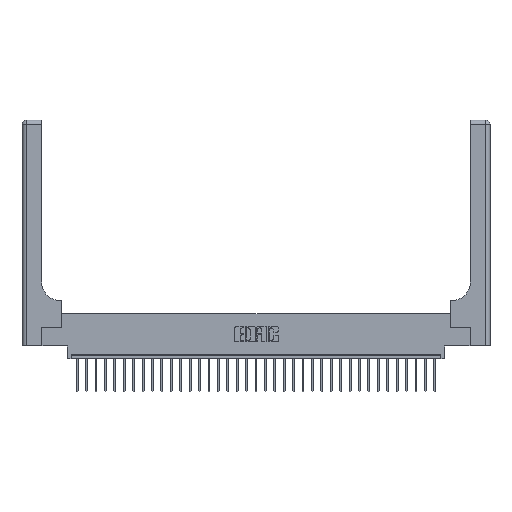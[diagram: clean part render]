
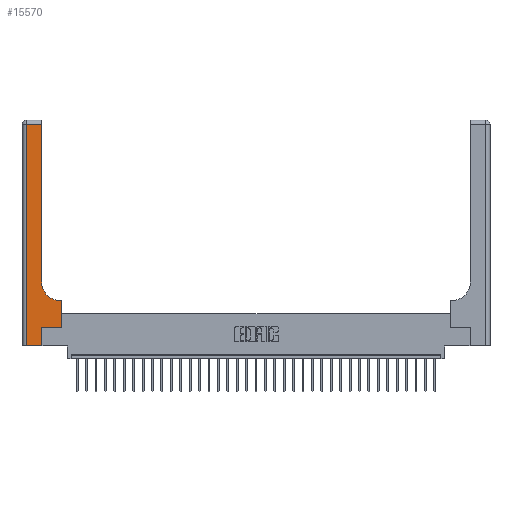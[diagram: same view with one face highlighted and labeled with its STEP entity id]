
A CAD part, top view. The second image highlights one B-rep face of the part: STEP entity #15570.
In plain terms, the highlighted planar face has unit normal (0, 0, 1).
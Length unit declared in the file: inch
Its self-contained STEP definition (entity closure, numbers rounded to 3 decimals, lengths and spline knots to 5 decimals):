
#124 = LINE ( 'NONE', #27338, #21756 ) ;
#267 = DIRECTION ( 'NONE',  ( 1., 0., 0. ) ) ;
#871 = DIRECTION ( 'NONE',  ( 0., 1., 0. ) ) ;
#1067 = ORIENTED_EDGE ( 'NONE', *, *, #16327, .T. ) ;
#2292 = CARTESIAN_POINT ( 'NONE',  ( 0.265, 0.25, 0.37 ) ) ;
#3273 = VECTOR ( 'NONE', #267, 39.37008 ) ;
#3409 = VECTOR ( 'NONE', #16758, 39.37008 ) ;
#4473 = LINE ( 'NONE', #23900, #3409 ) ;
#4961 = CARTESIAN_POINT ( 'NONE',  ( 0.26, 3., 0.37 ) ) ;
#4967 = VERTEX_POINT ( 'NONE', #17694 ) ;
#5303 = CARTESIAN_POINT ( 'NONE',  ( 0., 3., 0.37 ) ) ;
#5708 = DIRECTION ( 'NONE',  ( -1., 0., 0. ) ) ;
#6587 = CARTESIAN_POINT ( 'NONE',  ( 0.51, 0.6, 0.37 ) ) ;
#7037 = ORIENTED_EDGE ( 'NONE', *, *, #22949, .T. ) ;
#7261 = CARTESIAN_POINT ( 'NONE',  ( 0.265, 0., 0.37 ) ) ;
#7982 = VECTOR ( 'NONE', #13298, 39.37008 ) ;
#8178 = DIRECTION ( 'NONE',  ( 0., 0., -1. ) ) ;
#8664 = CARTESIAN_POINT ( 'NONE',  ( 0.528, 0.6, 0.37 ) ) ;
#9061 = ORIENTED_EDGE ( 'NONE', *, *, #29371, .T. ) ;
#9697 = VERTEX_POINT ( 'NONE', #9905 ) ;
#9905 = CARTESIAN_POINT ( 'NONE',  ( 0.06, 0., 0.37 ) ) ;
#10208 = CIRCLE ( 'NONE', #13667, 0.25 ) ;
#10263 = EDGE_CURVE ( 'NONE', #22879, #12880, #24050, .T. ) ;
#10901 = DIRECTION ( 'NONE',  ( 1., 0., 0. ) ) ;
#11764 = VECTOR ( 'NONE', #27981, 39.37008 ) ;
#11872 = EDGE_CURVE ( 'NONE', #21958, #19681, #124, .T. ) ;
#12359 = DIRECTION ( 'NONE',  ( 0., 0., -1. ) ) ;
#12382 = CARTESIAN_POINT ( 'NONE',  ( 0.26, 0.85, 0.37 ) ) ;
#12495 = VERTEX_POINT ( 'NONE', #7261 ) ;
#12880 = VERTEX_POINT ( 'NONE', #24333 ) ;
#13298 = DIRECTION ( 'NONE',  ( 0., 1., 0. ) ) ;
#13358 = ORIENTED_EDGE ( 'NONE', *, *, #26058, .T. ) ;
#13513 = DIRECTION ( 'NONE',  ( -1., 0., 0. ) ) ;
#13667 = AXIS2_PLACEMENT_3D ( 'NONE', #22011, #8178, #10901 ) ;
#13776 = EDGE_CURVE ( 'NONE', #16875, #22740, #24951, .T. ) ;
#14148 = LINE ( 'NONE', #29763, #7982 ) ;
#14664 = VECTOR ( 'NONE', #871, 39.37008 ) ;
#15029 = EDGE_LOOP ( 'NONE', ( #22875, #9061, #13358, #7037, #20525, #27619, #15866, #17852, #1067 ) ) ;
#15570 = ADVANCED_FACE ( 'NONE', ( #25421 ), #28629, .F. ) ;
#15866 = ORIENTED_EDGE ( 'NONE', *, *, #21366, .T. ) ;
#16327 = EDGE_CURVE ( 'NONE', #19681, #22879, #10208, .T. ) ;
#16538 = DIRECTION ( 'NONE',  ( 0., -1., 0. ) ) ;
#16758 = DIRECTION ( 'NONE',  ( 1., 0., 0. ) ) ;
#16875 = VERTEX_POINT ( 'NONE', #17321 ) ;
#17032 = VECTOR ( 'NONE', #16538, 39.37008 ) ;
#17145 = DIRECTION ( 'NONE',  ( -1., 0., 0. ) ) ;
#17321 = CARTESIAN_POINT ( 'NONE',  ( 0.265, 0.25, 0.37 ) ) ;
#17694 = CARTESIAN_POINT ( 'NONE',  ( 0.06, 2.94, 0.37 ) ) ;
#17852 = ORIENTED_EDGE ( 'NONE', *, *, #11872, .T. ) ;
#18104 = CARTESIAN_POINT ( 'NONE',  ( 0.528, 0.25, 0.37 ) ) ;
#19681 = VERTEX_POINT ( 'NONE', #6587 ) ;
#20041 = AXIS2_PLACEMENT_3D ( 'NONE', #5303, #12359, #17145 ) ;
#20525 = ORIENTED_EDGE ( 'NONE', *, *, #25707, .T. ) ;
#20837 = VECTOR ( 'NONE', #5708, 39.37008 ) ;
#21265 = CARTESIAN_POINT ( 'NONE',  ( 0.528, 0.25, 0.37 ) ) ;
#21366 = EDGE_CURVE ( 'NONE', #22740, #21958, #21839, .T. ) ;
#21756 = VECTOR ( 'NONE', #13513, 39.37008 ) ;
#21839 = LINE ( 'NONE', #21265, #14664 ) ;
#21958 = VERTEX_POINT ( 'NONE', #8664 ) ;
#22011 = CARTESIAN_POINT ( 'NONE',  ( 0.51, 0.85, 0.37 ) ) ;
#22740 = VERTEX_POINT ( 'NONE', #18104 ) ;
#22875 = ORIENTED_EDGE ( 'NONE', *, *, #10263, .T. ) ;
#22879 = VERTEX_POINT ( 'NONE', #12382 ) ;
#22949 = EDGE_CURVE ( 'NONE', #9697, #12495, #4473, .T. ) ;
#23138 = LINE ( 'NONE', #23785, #17032 ) ;
#23785 = CARTESIAN_POINT ( 'NONE',  ( 0.06, 3., 0.37 ) ) ;
#23900 = CARTESIAN_POINT ( 'NONE',  ( 0., 0., 0.37 ) ) ;
#24049 = LINE ( 'NONE', #26620, #20837 ) ;
#24050 = LINE ( 'NONE', #4961, #11764 ) ;
#24333 = CARTESIAN_POINT ( 'NONE',  ( 0.26, 2.94, 0.37 ) ) ;
#24951 = LINE ( 'NONE', #2292, #3273 ) ;
#25421 = FACE_OUTER_BOUND ( 'NONE', #15029, .T. ) ;
#25707 = EDGE_CURVE ( 'NONE', #12495, #16875, #14148, .T. ) ;
#26058 = EDGE_CURVE ( 'NONE', #4967, #9697, #23138, .T. ) ;
#26620 = CARTESIAN_POINT ( 'NONE',  ( 0., 2.94, 0.37 ) ) ;
#27338 = CARTESIAN_POINT ( 'NONE',  ( 0.26, 0.6, 0.37 ) ) ;
#27619 = ORIENTED_EDGE ( 'NONE', *, *, #13776, .T. ) ;
#27981 = DIRECTION ( 'NONE',  ( 0., 1., 0. ) ) ;
#28629 = PLANE ( 'NONE',  #20041 ) ;
#29371 = EDGE_CURVE ( 'NONE', #12880, #4967, #24049, .T. ) ;
#29763 = CARTESIAN_POINT ( 'NONE',  ( 0.265, 0., 0.37 ) ) ;
